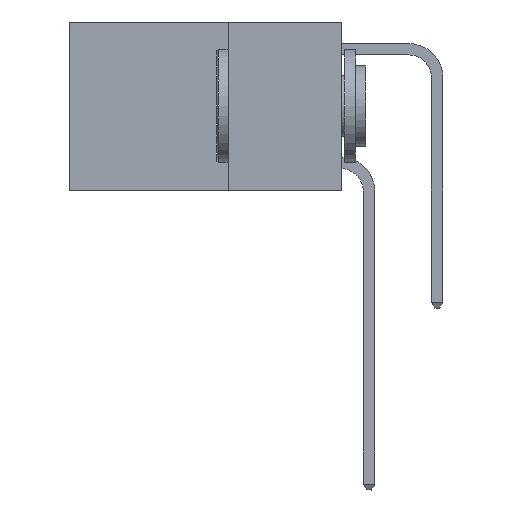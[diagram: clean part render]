
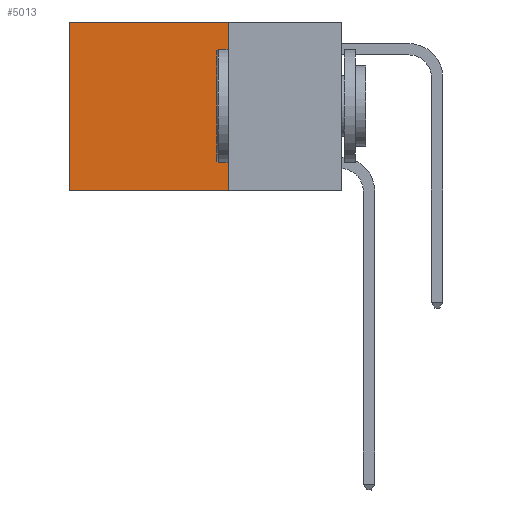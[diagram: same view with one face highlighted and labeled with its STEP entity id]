
A CAD part, left-side view. The second image highlights one B-rep face of the part: STEP entity #5013.
In plain terms, the highlighted planar face has unit normal (-1, 0, 0).
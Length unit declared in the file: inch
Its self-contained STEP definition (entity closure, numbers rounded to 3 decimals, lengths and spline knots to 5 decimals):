
#772 = DIRECTION ( 'NONE',  ( 0., 1., 0. ) ) ;
#818 = EDGE_CURVE ( 'NONE', #4405, #16135, #7488, .T. ) ;
#1160 = CARTESIAN_POINT ( 'NONE',  ( 0.2625, 0.6, 0. ) ) ;
#2645 = CARTESIAN_POINT ( 'NONE',  ( 0.2625, 0.25, 0. ) ) ;
#4405 = VERTEX_POINT ( 'NONE', #16855 ) ;
#5013 = ADVANCED_FACE ( 'NONE', ( #13442 ), #16680, .F. ) ;
#5527 = EDGE_LOOP ( 'NONE', ( #10998, #18218, #12137, #15222 ) ) ;
#6003 = DIRECTION ( 'NONE',  ( 0., 0., -1. ) ) ;
#7073 = VERTEX_POINT ( 'NONE', #10121 ) ;
#7181 = LINE ( 'NONE', #2645, #11433 ) ;
#7488 = LINE ( 'NONE', #17955, #21073 ) ;
#7504 = LINE ( 'NONE', #20247, #11723 ) ;
#9605 = DIRECTION ( 'NONE',  ( 0., 0., -1. ) ) ;
#10121 = CARTESIAN_POINT ( 'NONE',  ( 0.2625, 0.25, 0. ) ) ;
#10998 = ORIENTED_EDGE ( 'NONE', *, *, #12093, .T. ) ;
#11333 = VERTEX_POINT ( 'NONE', #16797 ) ;
#11433 = VECTOR ( 'NONE', #772, 39.37008 ) ;
#11440 = LINE ( 'NONE', #1160, #18377 ) ;
#11723 = VECTOR ( 'NONE', #6003, 39.37008 ) ;
#12093 = EDGE_CURVE ( 'NONE', #11333, #16135, #11440, .T. ) ;
#12137 = ORIENTED_EDGE ( 'NONE', *, *, #20072, .F. ) ;
#13050 = CARTESIAN_POINT ( 'NONE',  ( 0.2625, 0.6, -0.37 ) ) ;
#13124 = CARTESIAN_POINT ( 'NONE',  ( 0.2625, 0.25, 0. ) ) ;
#13442 = FACE_OUTER_BOUND ( 'NONE', #5527, .T. ) ;
#15197 = AXIS2_PLACEMENT_3D ( 'NONE', #13124, #20177, #9605 ) ;
#15222 = ORIENTED_EDGE ( 'NONE', *, *, #21053, .T. ) ;
#16135 = VERTEX_POINT ( 'NONE', #13050 ) ;
#16680 = PLANE ( 'NONE',  #15197 ) ;
#16797 = CARTESIAN_POINT ( 'NONE',  ( 0.2625, 0.6, 0. ) ) ;
#16855 = CARTESIAN_POINT ( 'NONE',  ( 0.2625, 0.25, -0.37 ) ) ;
#17955 = CARTESIAN_POINT ( 'NONE',  ( 0.2625, 0.25, -0.37 ) ) ;
#18083 = DIRECTION ( 'NONE',  ( 0., 1., 0. ) ) ;
#18218 = ORIENTED_EDGE ( 'NONE', *, *, #818, .F. ) ;
#18377 = VECTOR ( 'NONE', #19143, 39.37008 ) ;
#19143 = DIRECTION ( 'NONE',  ( 0., 0., -1. ) ) ;
#20072 = EDGE_CURVE ( 'NONE', #7073, #4405, #7504, .T. ) ;
#20177 = DIRECTION ( 'NONE',  ( 1., 0., 0. ) ) ;
#20247 = CARTESIAN_POINT ( 'NONE',  ( 0.2625, 0.25, 0. ) ) ;
#21053 = EDGE_CURVE ( 'NONE', #7073, #11333, #7181, .T. ) ;
#21073 = VECTOR ( 'NONE', #18083, 39.37008 ) ;
